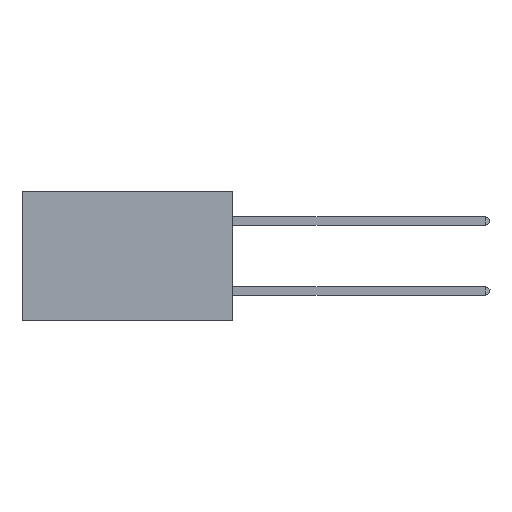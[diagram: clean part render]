
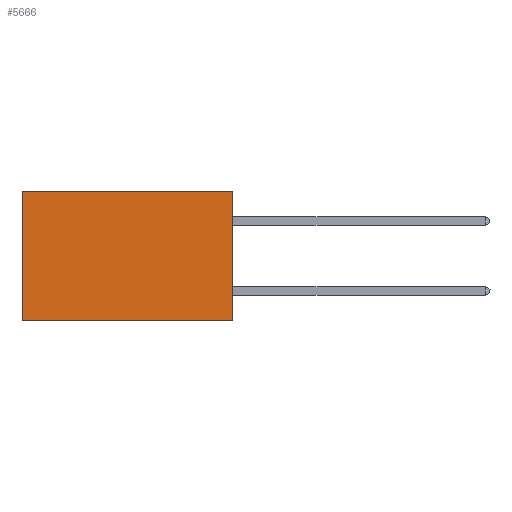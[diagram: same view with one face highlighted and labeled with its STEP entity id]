
A CAD part, left-side view. The second image highlights one B-rep face of the part: STEP entity #5666.
In plain terms, the highlighted planar face has unit normal (-1, 0, 0).
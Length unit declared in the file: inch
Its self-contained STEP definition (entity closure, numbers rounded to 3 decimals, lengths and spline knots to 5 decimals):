
#237 = CARTESIAN_POINT ( 'NONE',  ( 0.2875, 0., 0. ) ) ;
#459 = ORIENTED_EDGE ( 'NONE', *, *, #8061, .T. ) ;
#773 = EDGE_CURVE ( 'NONE', #4614, #11484, #8617, .T. ) ;
#1206 = DIRECTION ( 'NONE',  ( 0., 1., 0. ) ) ;
#1865 = VECTOR ( 'NONE', #7998, 39.37008 ) ;
#2373 = CARTESIAN_POINT ( 'NONE',  ( 0.2875, 0.6, 0. ) ) ;
#3241 = CARTESIAN_POINT ( 'NONE',  ( 0.2875, 0., -0.37 ) ) ;
#3612 = VECTOR ( 'NONE', #8848, 39.37008 ) ;
#3836 = CARTESIAN_POINT ( 'NONE',  ( 0.2875, 0.6, 0. ) ) ;
#3913 = DIRECTION ( 'NONE',  ( 0., 0., -1. ) ) ;
#4081 = CARTESIAN_POINT ( 'NONE',  ( 0.2875, 0., 0. ) ) ;
#4284 = EDGE_CURVE ( 'NONE', #11484, #9736, #4294, .T. ) ;
#4294 = LINE ( 'NONE', #3241, #1865 ) ;
#4498 = EDGE_CURVE ( 'NONE', #4614, #10519, #5485, .T. ) ;
#4614 = VERTEX_POINT ( 'NONE', #5119 ) ;
#5119 = CARTESIAN_POINT ( 'NONE',  ( 0.2875, 0., 0. ) ) ;
#5485 = LINE ( 'NONE', #4081, #9297 ) ;
#5666 = ADVANCED_FACE ( 'NONE', ( #6509 ), #6578, .F. ) ;
#5957 = ORIENTED_EDGE ( 'NONE', *, *, #773, .F. ) ;
#6509 = FACE_OUTER_BOUND ( 'NONE', #7790, .T. ) ;
#6578 = PLANE ( 'NONE',  #11239 ) ;
#6669 = CARTESIAN_POINT ( 'NONE',  ( 0.2875, 0.6, -0.37 ) ) ;
#7559 = DIRECTION ( 'NONE',  ( 1., 0., 0. ) ) ;
#7790 = EDGE_LOOP ( 'NONE', ( #459, #10958, #5957, #10532 ) ) ;
#7875 = CARTESIAN_POINT ( 'NONE',  ( 0.2875, 0., -0.37 ) ) ;
#7998 = DIRECTION ( 'NONE',  ( 0., 1., 0. ) ) ;
#8061 = EDGE_CURVE ( 'NONE', #10519, #9736, #11208, .T. ) ;
#8617 = LINE ( 'NONE', #237, #3612 ) ;
#8627 = VECTOR ( 'NONE', #3913, 39.37008 ) ;
#8848 = DIRECTION ( 'NONE',  ( 0., 0., -1. ) ) ;
#9297 = VECTOR ( 'NONE', #1206, 39.37008 ) ;
#9736 = VERTEX_POINT ( 'NONE', #6669 ) ;
#10476 = DIRECTION ( 'NONE',  ( 0., 0., -1. ) ) ;
#10519 = VERTEX_POINT ( 'NONE', #2373 ) ;
#10532 = ORIENTED_EDGE ( 'NONE', *, *, #4498, .T. ) ;
#10958 = ORIENTED_EDGE ( 'NONE', *, *, #4284, .F. ) ;
#11208 = LINE ( 'NONE', #3836, #8627 ) ;
#11239 = AXIS2_PLACEMENT_3D ( 'NONE', #12469, #7559, #10476 ) ;
#11484 = VERTEX_POINT ( 'NONE', #7875 ) ;
#12469 = CARTESIAN_POINT ( 'NONE',  ( 0.2875, 0., 0. ) ) ;
